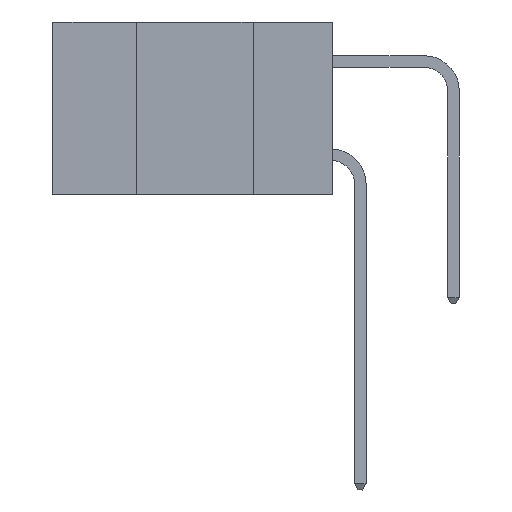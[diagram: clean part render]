
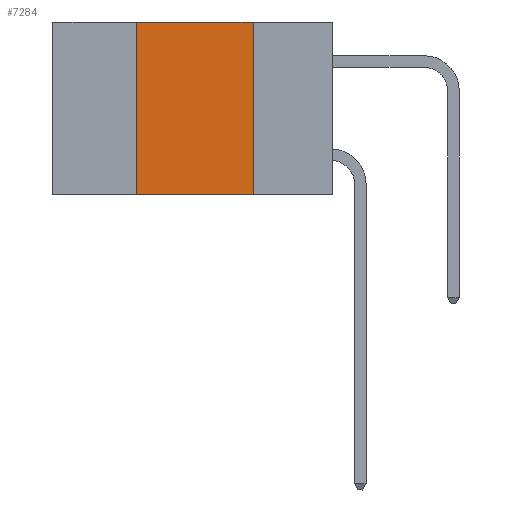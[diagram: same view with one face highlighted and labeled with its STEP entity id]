
A CAD part, left-side view. The second image highlights one B-rep face of the part: STEP entity #7284.
In plain terms, the highlighted planar face has unit normal (-1, 0, 0).
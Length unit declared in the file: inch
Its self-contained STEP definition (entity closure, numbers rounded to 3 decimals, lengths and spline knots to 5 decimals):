
#380 = VECTOR ( 'NONE', #12877, 39.37008 ) ;
#829 = EDGE_LOOP ( 'NONE', ( #12122, #8613, #9947, #9933 ) ) ;
#1495 = EDGE_CURVE ( 'NONE', #7021, #6540, #7507, .T. ) ;
#1855 = FACE_OUTER_BOUND ( 'NONE', #829, .T. ) ;
#1893 = CARTESIAN_POINT ( 'NONE',  ( 0., 0.6, 0. ) ) ;
#1896 = LINE ( 'NONE', #7708, #16483 ) ;
#2125 = DIRECTION ( 'NONE',  ( 0., -1., 0. ) ) ;
#3634 = EDGE_CURVE ( 'NONE', #9848, #12111, #7236, .T. ) ;
#3797 = VECTOR ( 'NONE', #10584, 39.37008 ) ;
#4300 = CARTESIAN_POINT ( 'NONE',  ( 0., 0.17, 0. ) ) ;
#5605 = PLANE ( 'NONE',  #10137 ) ;
#6087 = LINE ( 'NONE', #1893, #12996 ) ;
#6376 = CARTESIAN_POINT ( 'NONE',  ( 0., 0.17, 0. ) ) ;
#6540 = VERTEX_POINT ( 'NONE', #15750 ) ;
#7019 = DIRECTION ( 'NONE',  ( 0., 0., -1. ) ) ;
#7021 = VERTEX_POINT ( 'NONE', #6376 ) ;
#7236 = LINE ( 'NONE', #12394, #380 ) ;
#7284 = ADVANCED_FACE ( 'NONE', ( #1855 ), #5605, .F. ) ;
#7507 = LINE ( 'NONE', #4300, #3797 ) ;
#7708 = CARTESIAN_POINT ( 'NONE',  ( 0., 0.6, -0.37 ) ) ;
#8613 = ORIENTED_EDGE ( 'NONE', *, *, #9429, .F. ) ;
#9429 = EDGE_CURVE ( 'NONE', #12111, #7021, #6087, .T. ) ;
#9848 = VERTEX_POINT ( 'NONE', #16412 ) ;
#9933 = ORIENTED_EDGE ( 'NONE', *, *, #15083, .T. ) ;
#9947 = ORIENTED_EDGE ( 'NONE', *, *, #3634, .F. ) ;
#10137 = AXIS2_PLACEMENT_3D ( 'NONE', #11590, #15246, #7019 ) ;
#10584 = DIRECTION ( 'NONE',  ( 0., 0., -1. ) ) ;
#11590 = CARTESIAN_POINT ( 'NONE',  ( 0., 0.6, 0. ) ) ;
#12111 = VERTEX_POINT ( 'NONE', #15713 ) ;
#12122 = ORIENTED_EDGE ( 'NONE', *, *, #1495, .F. ) ;
#12394 = CARTESIAN_POINT ( 'NONE',  ( 0., 0.42, 0. ) ) ;
#12877 = DIRECTION ( 'NONE',  ( 0., 0., 1. ) ) ;
#12996 = VECTOR ( 'NONE', #2125, 39.37008 ) ;
#15083 = EDGE_CURVE ( 'NONE', #9848, #6540, #1896, .T. ) ;
#15246 = DIRECTION ( 'NONE',  ( 1., 0., 0. ) ) ;
#15713 = CARTESIAN_POINT ( 'NONE',  ( 0., 0.42, 0. ) ) ;
#15750 = CARTESIAN_POINT ( 'NONE',  ( 0., 0.17, -0.37 ) ) ;
#16412 = CARTESIAN_POINT ( 'NONE',  ( 0., 0.42, -0.37 ) ) ;
#16483 = VECTOR ( 'NONE', #17251, 39.37008 ) ;
#17251 = DIRECTION ( 'NONE',  ( 0., -1., 0. ) ) ;
